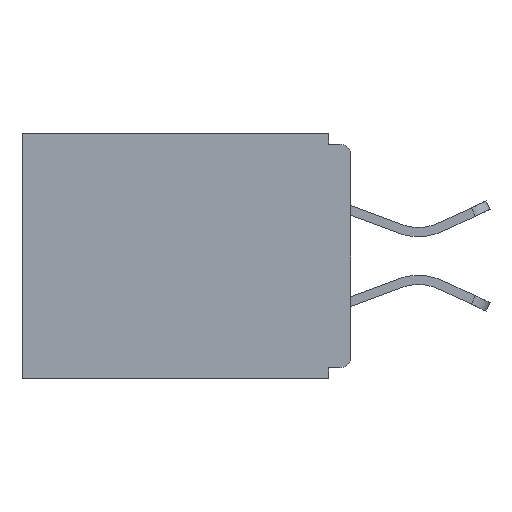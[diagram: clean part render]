
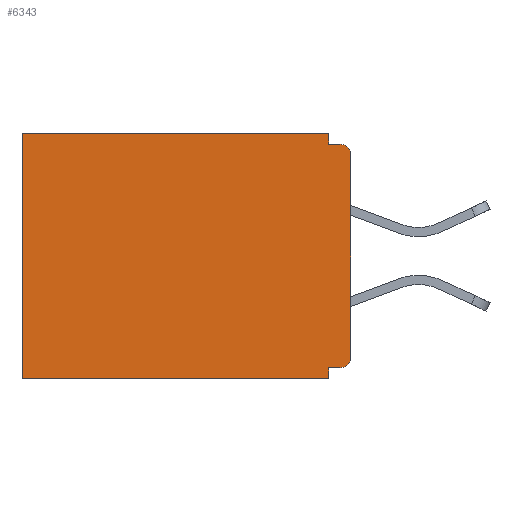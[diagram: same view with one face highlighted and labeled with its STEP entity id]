
A CAD part, left-side view. The second image highlights one B-rep face of the part: STEP entity #6343.
In plain terms, the highlighted planar face has unit normal (-1, 0, 0).
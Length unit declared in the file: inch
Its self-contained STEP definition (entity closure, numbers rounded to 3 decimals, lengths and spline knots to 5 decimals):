
#161 = LINE ( 'NONE', #13861, #6591 ) ;
#164 = DIRECTION ( 'NONE',  ( 1., 0., 0. ) ) ;
#211 = CARTESIAN_POINT ( 'NONE',  ( 0.298, 0.031, -0.015 ) ) ;
#250 = EDGE_LOOP ( 'NONE', ( #20311, #17399, #9096, #8935, #15775, #14343, #15068, #18217, #18482, #17142 ) ) ;
#253 = VECTOR ( 'NONE', #12698, 39.37008 ) ;
#261 = DIRECTION ( 'NONE',  ( 0., 0., -1. ) ) ;
#468 = VERTEX_POINT ( 'NONE', #19900 ) ;
#505 = EDGE_CURVE ( 'NONE', #468, #10366, #11505, .T. ) ;
#661 = VERTEX_POINT ( 'NONE', #19074 ) ;
#1175 = DIRECTION ( 'NONE',  ( 0., 0., -1. ) ) ;
#1840 = VECTOR ( 'NONE', #1175, 39.37008 ) ;
#2312 = VECTOR ( 'NONE', #11587, 39.37008 ) ;
#2420 = VERTEX_POINT ( 'NONE', #17006 ) ;
#2601 = AXIS2_PLACEMENT_3D ( 'NONE', #6139, #4893, #261 ) ;
#2676 = CARTESIAN_POINT ( 'NONE',  ( 0.298, 0.031, -0.343 ) ) ;
#2894 = LINE ( 'NONE', #15497, #17190 ) ;
#2998 = VERTEX_POINT ( 'NONE', #211 ) ;
#4391 = VERTEX_POINT ( 'NONE', #18687 ) ;
#4589 = DIRECTION ( 'NONE',  ( 0., 0., -1. ) ) ;
#4630 = VERTEX_POINT ( 'NONE', #15981 ) ;
#4734 = DIRECTION ( 'NONE',  ( 0., 0., -1. ) ) ;
#4865 = EDGE_CURVE ( 'NONE', #8368, #4630, #17310, .T. ) ;
#4893 = DIRECTION ( 'NONE',  ( -1., 0., 0. ) ) ;
#4992 = CARTESIAN_POINT ( 'NONE',  ( 0.298, 0.015, -0.313 ) ) ;
#5249 = LINE ( 'NONE', #5827, #16335 ) ;
#5544 = LINE ( 'NONE', #14710, #2312 ) ;
#5827 = CARTESIAN_POINT ( 'NONE',  ( 0.298, 0., -0.015 ) ) ;
#6016 = EDGE_CURVE ( 'NONE', #13559, #661, #2894, .T. ) ;
#6046 = DIRECTION ( 'NONE',  ( 0., 1., 0. ) ) ;
#6139 = CARTESIAN_POINT ( 'NONE',  ( 0.298, 0.015, -0.03 ) ) ;
#6171 = CARTESIAN_POINT ( 'NONE',  ( 0.298, 0., -0.328 ) ) ;
#6336 = DIRECTION ( 'NONE',  ( 0., 1., 0. ) ) ;
#6343 = ADVANCED_FACE ( 'NONE', ( #16469 ), #14202, .F. ) ;
#6448 = DIRECTION ( 'NONE',  ( -1., 0., 0. ) ) ;
#6591 = VECTOR ( 'NONE', #4589, 39.37008 ) ;
#7343 = LINE ( 'NONE', #2676, #1840 ) ;
#7770 = DIRECTION ( 'NONE',  ( 0., 1., 0. ) ) ;
#8311 = VERTEX_POINT ( 'NONE', #9022 ) ;
#8368 = VERTEX_POINT ( 'NONE', #12052 ) ;
#8935 = ORIENTED_EDGE ( 'NONE', *, *, #505, .T. ) ;
#9022 = CARTESIAN_POINT ( 'NONE',  ( 0.298, 0., -0.03 ) ) ;
#9096 = ORIENTED_EDGE ( 'NONE', *, *, #18000, .F. ) ;
#9117 = EDGE_CURVE ( 'NONE', #2998, #2420, #5249, .T. ) ;
#10022 = EDGE_CURVE ( 'NONE', #10366, #661, #19767, .T. ) ;
#10366 = VERTEX_POINT ( 'NONE', #15759 ) ;
#10518 = AXIS2_PLACEMENT_3D ( 'NONE', #4992, #6448, #4734 ) ;
#11283 = VECTOR ( 'NONE', #6046, 39.37008 ) ;
#11505 = LINE ( 'NONE', #13670, #11283 ) ;
#11587 = DIRECTION ( 'NONE',  ( 0., 0., -1. ) ) ;
#12052 = CARTESIAN_POINT ( 'NONE',  ( 0.298, 0.015, -0.328 ) ) ;
#12698 = DIRECTION ( 'NONE',  ( 0., 0., -1. ) ) ;
#13058 = EDGE_CURVE ( 'NONE', #8368, #4391, #18099, .T. ) ;
#13559 = VERTEX_POINT ( 'NONE', #17783 ) ;
#13670 = CARTESIAN_POINT ( 'NONE',  ( 0.298, 0., 0. ) ) ;
#13861 = CARTESIAN_POINT ( 'NONE',  ( 0.298, 0., 0. ) ) ;
#14071 = VECTOR ( 'NONE', #7770, 39.37008 ) ;
#14202 = PLANE ( 'NONE',  #16218 ) ;
#14343 = ORIENTED_EDGE ( 'NONE', *, *, #6016, .F. ) ;
#14477 = DIRECTION ( 'NONE',  ( 0., 0., -1. ) ) ;
#14710 = CARTESIAN_POINT ( 'NONE',  ( 0.298, 0.031, -0.343 ) ) ;
#15068 = ORIENTED_EDGE ( 'NONE', *, *, #18936, .F. ) ;
#15497 = CARTESIAN_POINT ( 'NONE',  ( 0.298, 0., -0.343 ) ) ;
#15575 = DIRECTION ( 'NONE',  ( 0., -1., 0. ) ) ;
#15695 = EDGE_CURVE ( 'NONE', #8311, #2420, #16919, .T. ) ;
#15759 = CARTESIAN_POINT ( 'NONE',  ( 0.298, 0.46, 0. ) ) ;
#15775 = ORIENTED_EDGE ( 'NONE', *, *, #10022, .T. ) ;
#15981 = CARTESIAN_POINT ( 'NONE',  ( 0.298, 0., -0.313 ) ) ;
#16218 = AXIS2_PLACEMENT_3D ( 'NONE', #19072, #164, #14477 ) ;
#16335 = VECTOR ( 'NONE', #15575, 39.37008 ) ;
#16469 = FACE_OUTER_BOUND ( 'NONE', #250, .T. ) ;
#16745 = EDGE_CURVE ( 'NONE', #8311, #4630, #161, .T. ) ;
#16919 = CIRCLE ( 'NONE', #2601, 0.015 ) ;
#17006 = CARTESIAN_POINT ( 'NONE',  ( 0.298, 0.015, -0.015 ) ) ;
#17142 = ORIENTED_EDGE ( 'NONE', *, *, #16745, .F. ) ;
#17190 = VECTOR ( 'NONE', #6336, 39.37008 ) ;
#17310 = CIRCLE ( 'NONE', #10518, 0.015 ) ;
#17399 = ORIENTED_EDGE ( 'NONE', *, *, #9117, .F. ) ;
#17783 = CARTESIAN_POINT ( 'NONE',  ( 0.298, 0.031, -0.343 ) ) ;
#18000 = EDGE_CURVE ( 'NONE', #468, #2998, #7343, .T. ) ;
#18099 = LINE ( 'NONE', #6171, #14071 ) ;
#18217 = ORIENTED_EDGE ( 'NONE', *, *, #13058, .F. ) ;
#18482 = ORIENTED_EDGE ( 'NONE', *, *, #4865, .T. ) ;
#18687 = CARTESIAN_POINT ( 'NONE',  ( 0.298, 0.031, -0.328 ) ) ;
#18936 = EDGE_CURVE ( 'NONE', #4391, #13559, #5544, .T. ) ;
#19072 = CARTESIAN_POINT ( 'NONE',  ( 0.298, 0., 0. ) ) ;
#19074 = CARTESIAN_POINT ( 'NONE',  ( 0.298, 0.46, -0.343 ) ) ;
#19767 = LINE ( 'NONE', #20244, #253 ) ;
#19900 = CARTESIAN_POINT ( 'NONE',  ( 0.298, 0.031, 0. ) ) ;
#20244 = CARTESIAN_POINT ( 'NONE',  ( 0.298, 0.46, 0. ) ) ;
#20311 = ORIENTED_EDGE ( 'NONE', *, *, #15695, .T. ) ;
